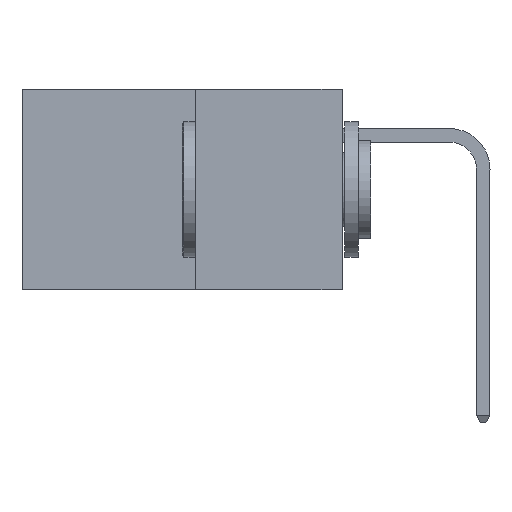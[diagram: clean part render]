
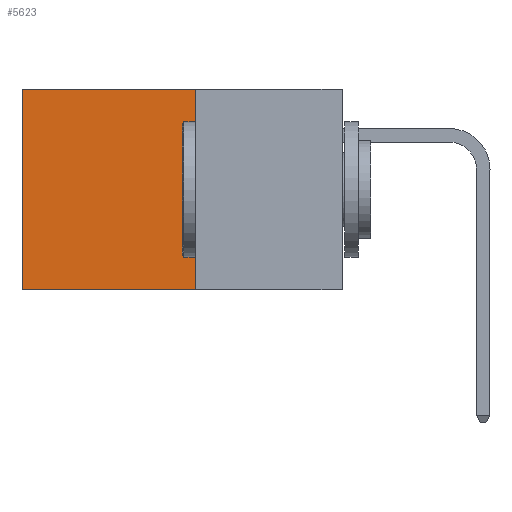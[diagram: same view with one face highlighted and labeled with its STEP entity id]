
A CAD part, left-side view. The second image highlights one B-rep face of the part: STEP entity #5623.
In plain terms, the highlighted planar face has unit normal (-1, 0, 0).
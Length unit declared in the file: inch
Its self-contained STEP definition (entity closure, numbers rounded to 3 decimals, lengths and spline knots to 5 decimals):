
#281 = CARTESIAN_POINT ( 'NONE',  ( 0.277, 0.27, -0.37 ) ) ;
#1096 = VECTOR ( 'NONE', #10215, 39.37008 ) ;
#1700 = FACE_OUTER_BOUND ( 'NONE', #20766, .T. ) ;
#1774 = CARTESIAN_POINT ( 'NONE',  ( 0.277, 0.27, -0.37 ) ) ;
#2550 = CARTESIAN_POINT ( 'NONE',  ( 0.277, 0.27, 0. ) ) ;
#3004 = CARTESIAN_POINT ( 'NONE',  ( 0.277, 0.27, 0. ) ) ;
#3310 = EDGE_CURVE ( 'NONE', #21071, #19841, #18594, .T. ) ;
#3425 = VERTEX_POINT ( 'NONE', #2550 ) ;
#4845 = EDGE_CURVE ( 'NONE', #23387, #19841, #20945, .T. ) ;
#5158 = CARTESIAN_POINT ( 'NONE',  ( 0.277, 0.59, 0. ) ) ;
#5546 = DIRECTION ( 'NONE',  ( 0., 0., -1. ) ) ;
#5623 = ADVANCED_FACE ( 'NONE', ( #1700 ), #5894, .F. ) ;
#5625 = DIRECTION ( 'NONE',  ( 1., 0., 0. ) ) ;
#5660 = CARTESIAN_POINT ( 'NONE',  ( 0.277, 0.27, -0.37 ) ) ;
#5894 = PLANE ( 'NONE',  #10472 ) ;
#6873 = CARTESIAN_POINT ( 'NONE',  ( 0.277, 0.59, -0.37 ) ) ;
#6891 = ORIENTED_EDGE ( 'NONE', *, *, #4845, .T. ) ;
#10215 = DIRECTION ( 'NONE',  ( 0., 1., 0. ) ) ;
#10472 = AXIS2_PLACEMENT_3D ( 'NONE', #5660, #5625, #5546 ) ;
#10622 = VECTOR ( 'NONE', #20256, 39.37008 ) ;
#10705 = EDGE_CURVE ( 'NONE', #3425, #23387, #20905, .T. ) ;
#10951 = VECTOR ( 'NONE', #22109, 39.37008 ) ;
#11480 = ORIENTED_EDGE ( 'NONE', *, *, #3310, .F. ) ;
#13791 = VECTOR ( 'NONE', #13864, 39.37008 ) ;
#13864 = DIRECTION ( 'NONE',  ( 0., 1., 0. ) ) ;
#14208 = ORIENTED_EDGE ( 'NONE', *, *, #10705, .T. ) ;
#16307 = EDGE_CURVE ( 'NONE', #3425, #21071, #19542, .T. ) ;
#18594 = LINE ( 'NONE', #1774, #13791 ) ;
#19542 = LINE ( 'NONE', #281, #10622 ) ;
#19841 = VERTEX_POINT ( 'NONE', #6873 ) ;
#20256 = DIRECTION ( 'NONE',  ( 0., 0., -1. ) ) ;
#20766 = EDGE_LOOP ( 'NONE', ( #6891, #11480, #22236, #14208 ) ) ;
#20905 = LINE ( 'NONE', #3004, #1096 ) ;
#20945 = LINE ( 'NONE', #21925, #10951 ) ;
#21071 = VERTEX_POINT ( 'NONE', #23164 ) ;
#21925 = CARTESIAN_POINT ( 'NONE',  ( 0.277, 0.59, -0.37 ) ) ;
#22109 = DIRECTION ( 'NONE',  ( 0., 0., -1. ) ) ;
#22236 = ORIENTED_EDGE ( 'NONE', *, *, #16307, .F. ) ;
#23164 = CARTESIAN_POINT ( 'NONE',  ( 0.277, 0.27, -0.37 ) ) ;
#23387 = VERTEX_POINT ( 'NONE', #5158 ) ;
